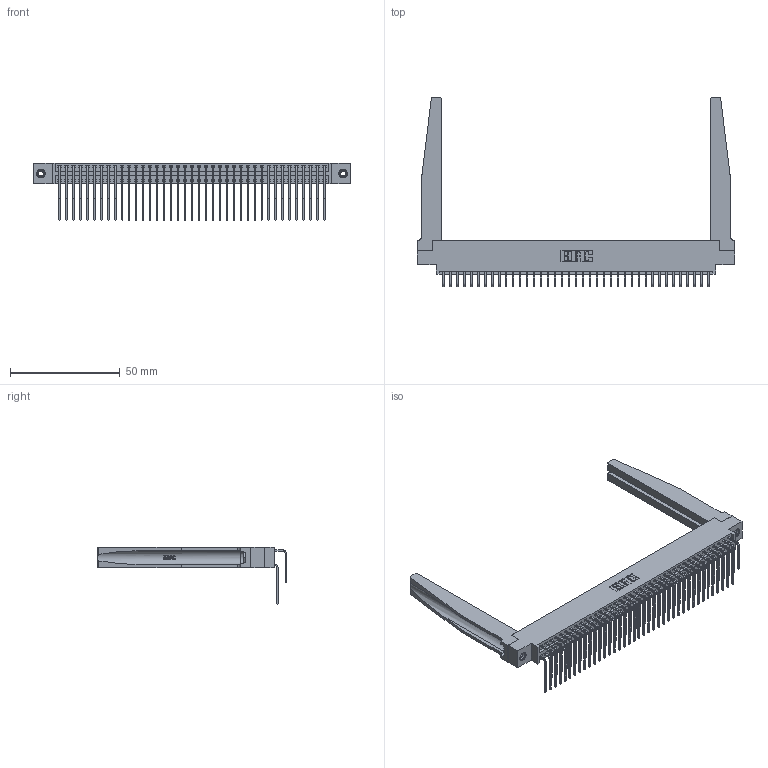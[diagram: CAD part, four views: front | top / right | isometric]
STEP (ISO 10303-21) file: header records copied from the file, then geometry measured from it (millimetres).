
FILE_DESCRIPTION (( 'STEP AP203' ), '1' );
FILE_NAME ('396-078-559-878.STEP', '2019-11-03T12:31:49', ( '' ), ( '' ), 'SwSTEP 2.0', 'SolidWorks 2016', '' );
FILE_SCHEMA (( 'CONFIG_CONTROL_DESIGN' ));
Length unit declared in the file: inch
Products named in the file (6): 345-292-001_559 Tail - 2; 345-292-001_558 559 Tail - 1; 346-220-078_345-220-078; 345-250-001_345-250-001-102; 346 Part_0.170 Offset - 0.156 Dia-TH; 396-078-559-878
Assembly tree (83 placements, depth 2):
  396-078-559-878
    346 Part_0.170 Offset - 0.156 Dia-TH
    345-292-001_558 559 Tail - 1  x39
    345-292-001_559 Tail - 2  x39
    346-220-078_345-220-078  x2
    345-250-001_345-250-001-102  x2
Bounding box: 144.4 x 86.17 x 26.16 mm (x, y, z)
Volume: 21261.6 mm3; surface area: 28557.4 mm2
Topology: 83 solids, 83 shells, 4572 faces, 13507 edges, 8890 vertices
Faces by surface type: plane 3108, cylinder 1412, bspline 36, cone 12, torus 4
Entity records: 32520 total; most frequent: CARTESIAN_POINT 6354, ORIENTED_EDGE 5126, DIRECTION 4609, EDGE_CURVE 2563, VECTOR 2141, LINE 2141, VERTEX_POINT 1700, AXIS2_PLACEMENT_3D 1234
